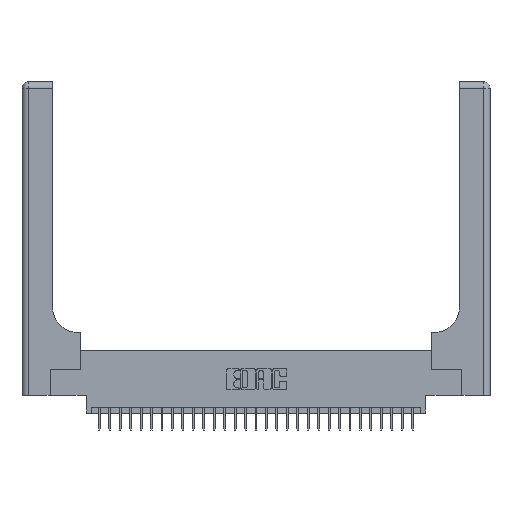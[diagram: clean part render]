
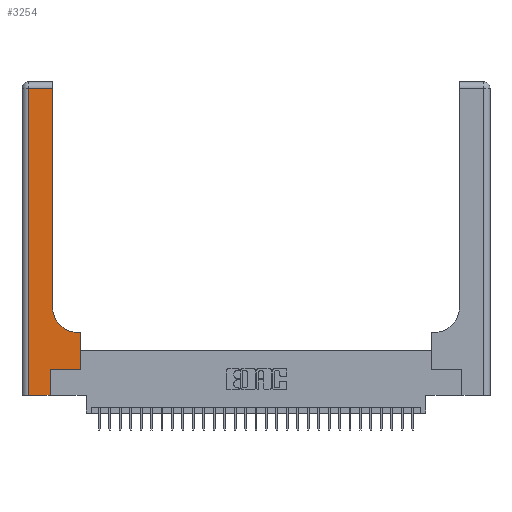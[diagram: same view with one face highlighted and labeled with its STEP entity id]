
A CAD part, top view. The second image highlights one B-rep face of the part: STEP entity #3254.
In plain terms, the highlighted planar face has unit normal (0, 0, 1).
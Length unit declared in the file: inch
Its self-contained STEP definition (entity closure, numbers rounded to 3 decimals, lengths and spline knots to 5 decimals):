
#293 = ORIENTED_EDGE ( 'NONE', *, *, #19606, .T. ) ;
#800 = CARTESIAN_POINT ( 'NONE',  ( 0.5415, 0.85, 0.37 ) ) ;
#1243 = EDGE_LOOP ( 'NONE', ( #10253, #8057, #17184, #16007, #293, #14352, #22826, #24393, #5567 ) ) ;
#2108 = DIRECTION ( 'NONE',  ( 0., 0., -1. ) ) ;
#3232 = CARTESIAN_POINT ( 'NONE',  ( 0., 0., 0.37 ) ) ;
#3254 = ADVANCED_FACE ( 'NONE', ( #28665 ), #23754, .F. ) ;
#3326 = CARTESIAN_POINT ( 'NONE',  ( 0.269, 0., 0.37 ) ) ;
#3639 = LINE ( 'NONE', #21445, #13066 ) ;
#4083 = CIRCLE ( 'NONE', #24466, 0.25 ) ;
#4206 = VERTEX_POINT ( 'NONE', #15960 ) ;
#5017 = LINE ( 'NONE', #24780, #9177 ) ;
#5533 = DIRECTION ( 'NONE',  ( 1., 0., 0. ) ) ;
#5540 = DIRECTION ( 'NONE',  ( 1., 0., 0. ) ) ;
#5567 = ORIENTED_EDGE ( 'NONE', *, *, #19487, .T. ) ;
#6439 = EDGE_CURVE ( 'NONE', #29047, #12003, #5017, .T. ) ;
#6723 = DIRECTION ( 'NONE',  ( -1., 0., 0. ) ) ;
#6944 = CARTESIAN_POINT ( 'NONE',  ( 0., 3., 0.37 ) ) ;
#7187 = EDGE_CURVE ( 'NONE', #4206, #19964, #25428, .T. ) ;
#7443 = DIRECTION ( 'NONE',  ( 0., 1., 0. ) ) ;
#7647 = CARTESIAN_POINT ( 'NONE',  ( 0.269, 0.25, 0.37 ) ) ;
#7943 = LINE ( 'NONE', #18764, #14375 ) ;
#8057 = ORIENTED_EDGE ( 'NONE', *, *, #20568, .T. ) ;
#8388 = CARTESIAN_POINT ( 'NONE',  ( 0.2915, 3., 0.37 ) ) ;
#8505 = DIRECTION ( 'NONE',  ( 0., 1., 0. ) ) ;
#9177 = VECTOR ( 'NONE', #7443, 39.37008 ) ;
#9328 = CARTESIAN_POINT ( 'NONE',  ( 0.5585, 0.6, 0.37 ) ) ;
#9616 = EDGE_CURVE ( 'NONE', #12003, #28931, #20296, .T. ) ;
#9755 = CARTESIAN_POINT ( 'NONE',  ( 0.2915, 2.94, 0.37 ) ) ;
#9858 = VERTEX_POINT ( 'NONE', #9755 ) ;
#9966 = VERTEX_POINT ( 'NONE', #16424 ) ;
#10253 = ORIENTED_EDGE ( 'NONE', *, *, #10647, .T. ) ;
#10647 = EDGE_CURVE ( 'NONE', #9966, #9858, #15292, .T. ) ;
#11580 = DIRECTION ( 'NONE',  ( 0., -1., 0. ) ) ;
#12003 = VERTEX_POINT ( 'NONE', #9328 ) ;
#12809 = AXIS2_PLACEMENT_3D ( 'NONE', #6944, #2108, #6723 ) ;
#12828 = DIRECTION ( 'NONE',  ( 0., 0., -1. ) ) ;
#12945 = VECTOR ( 'NONE', #21928, 39.37008 ) ;
#12969 = VECTOR ( 'NONE', #5540, 39.37008 ) ;
#13066 = VECTOR ( 'NONE', #28693, 39.37008 ) ;
#13125 = LINE ( 'NONE', #3326, #22212 ) ;
#13491 = VERTEX_POINT ( 'NONE', #20942 ) ;
#14143 = EDGE_CURVE ( 'NONE', #29280, #4206, #7943, .T. ) ;
#14352 = ORIENTED_EDGE ( 'NONE', *, *, #16916, .T. ) ;
#14375 = VECTOR ( 'NONE', #11580, 39.37008 ) ;
#14545 = DIRECTION ( 'NONE',  ( -1., 0., 0. ) ) ;
#14781 = CARTESIAN_POINT ( 'NONE',  ( 0.269, 0., 0.37 ) ) ;
#14922 = VECTOR ( 'NONE', #22755, 39.37008 ) ;
#15292 = LINE ( 'NONE', #8388, #14922 ) ;
#15960 = CARTESIAN_POINT ( 'NONE',  ( 0.06, 0., 0.37 ) ) ;
#16007 = ORIENTED_EDGE ( 'NONE', *, *, #7187, .T. ) ;
#16424 = CARTESIAN_POINT ( 'NONE',  ( 0.2915, 0.85, 0.37 ) ) ;
#16832 = CARTESIAN_POINT ( 'NONE',  ( 0.2915, 0.6, 0.37 ) ) ;
#16916 = EDGE_CURVE ( 'NONE', #13491, #29047, #17818, .T. ) ;
#17184 = ORIENTED_EDGE ( 'NONE', *, *, #14143, .T. ) ;
#17539 = CARTESIAN_POINT ( 'NONE',  ( 0.06, 2.94, 0.37 ) ) ;
#17818 = LINE ( 'NONE', #7647, #12945 ) ;
#18640 = CARTESIAN_POINT ( 'NONE',  ( 0.5415, 0.6, 0.37 ) ) ;
#18764 = CARTESIAN_POINT ( 'NONE',  ( 0.06, 3., 0.37 ) ) ;
#19487 = EDGE_CURVE ( 'NONE', #28931, #9966, #4083, .T. ) ;
#19606 = EDGE_CURVE ( 'NONE', #19964, #13491, #13125, .T. ) ;
#19964 = VERTEX_POINT ( 'NONE', #14781 ) ;
#20296 = LINE ( 'NONE', #16832, #24454 ) ;
#20568 = EDGE_CURVE ( 'NONE', #9858, #29280, #3639, .T. ) ;
#20942 = CARTESIAN_POINT ( 'NONE',  ( 0.269, 0.25, 0.37 ) ) ;
#21445 = CARTESIAN_POINT ( 'NONE',  ( 0., 2.94, 0.37 ) ) ;
#21928 = DIRECTION ( 'NONE',  ( 1., 0., 0. ) ) ;
#22212 = VECTOR ( 'NONE', #8505, 39.37008 ) ;
#22755 = DIRECTION ( 'NONE',  ( 0., 1., 0. ) ) ;
#22826 = ORIENTED_EDGE ( 'NONE', *, *, #6439, .T. ) ;
#23754 = PLANE ( 'NONE',  #12809 ) ;
#24393 = ORIENTED_EDGE ( 'NONE', *, *, #9616, .T. ) ;
#24454 = VECTOR ( 'NONE', #14545, 39.37008 ) ;
#24466 = AXIS2_PLACEMENT_3D ( 'NONE', #800, #12828, #5533 ) ;
#24780 = CARTESIAN_POINT ( 'NONE',  ( 0.5585, 0.25, 0.37 ) ) ;
#25428 = LINE ( 'NONE', #3232, #12969 ) ;
#26668 = CARTESIAN_POINT ( 'NONE',  ( 0.5585, 0.25, 0.37 ) ) ;
#28665 = FACE_OUTER_BOUND ( 'NONE', #1243, .T. ) ;
#28693 = DIRECTION ( 'NONE',  ( -1., 0., 0. ) ) ;
#28931 = VERTEX_POINT ( 'NONE', #18640 ) ;
#29047 = VERTEX_POINT ( 'NONE', #26668 ) ;
#29280 = VERTEX_POINT ( 'NONE', #17539 ) ;
